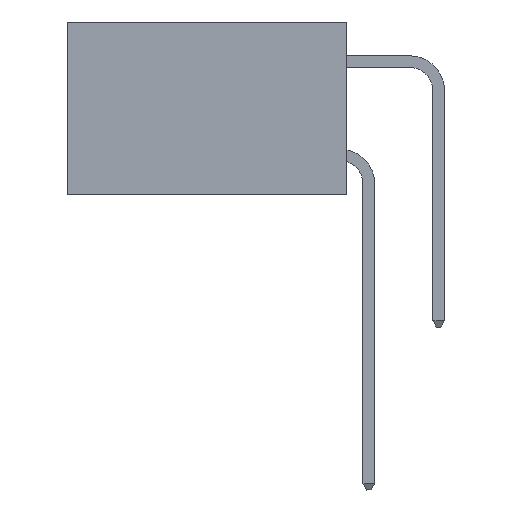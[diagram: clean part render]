
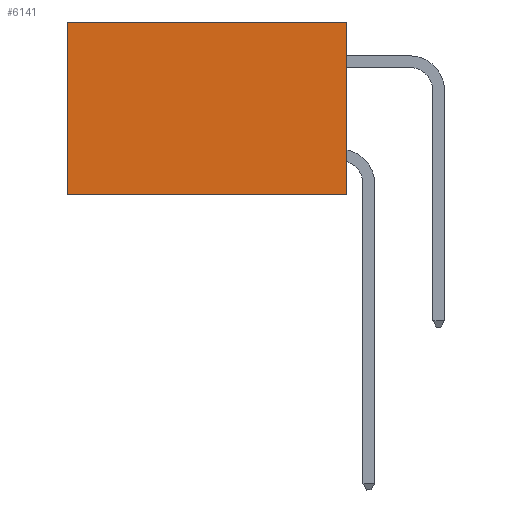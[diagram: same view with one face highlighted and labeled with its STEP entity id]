
A CAD part, left-side view. The second image highlights one B-rep face of the part: STEP entity #6141.
In plain terms, the highlighted planar face has unit normal (-1, 0, 0).
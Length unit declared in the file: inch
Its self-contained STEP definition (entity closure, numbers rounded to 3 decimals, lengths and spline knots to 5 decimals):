
#54 = DIRECTION ( 'NONE',  ( 0., 1., 0. ) ) ;
#268 = CARTESIAN_POINT ( 'NONE',  ( 0.2875, 0., 0. ) ) ;
#1064 = LINE ( 'NONE', #1661, #9241 ) ;
#1231 = AXIS2_PLACEMENT_3D ( 'NONE', #5987, #2249, #14703 ) ;
#1247 = ORIENTED_EDGE ( 'NONE', *, *, #15911, .F. ) ;
#1661 = CARTESIAN_POINT ( 'NONE',  ( 0.2875, 0., -0.37 ) ) ;
#1924 = VERTEX_POINT ( 'NONE', #8325 ) ;
#1975 = ORIENTED_EDGE ( 'NONE', *, *, #13054, .T. ) ;
#2249 = DIRECTION ( 'NONE',  ( 1., 0., 0. ) ) ;
#3926 = VERTEX_POINT ( 'NONE', #13418 ) ;
#4252 = EDGE_LOOP ( 'NONE', ( #5219, #1247, #13657, #1975 ) ) ;
#4664 = PLANE ( 'NONE',  #1231 ) ;
#4826 = EDGE_CURVE ( 'NONE', #14989, #8077, #6170, .T. ) ;
#4988 = FACE_OUTER_BOUND ( 'NONE', #4252, .T. ) ;
#5208 = EDGE_CURVE ( 'NONE', #3926, #1924, #13408, .T. ) ;
#5219 = ORIENTED_EDGE ( 'NONE', *, *, #5208, .T. ) ;
#5987 = CARTESIAN_POINT ( 'NONE',  ( 0.2875, 0., 0. ) ) ;
#6141 = ADVANCED_FACE ( 'NONE', ( #4988 ), #4664, .F. ) ;
#6170 = LINE ( 'NONE', #10400, #11237 ) ;
#6533 = DIRECTION ( 'NONE',  ( 0., 0., -1. ) ) ;
#6635 = LINE ( 'NONE', #268, #9343 ) ;
#8077 = VERTEX_POINT ( 'NONE', #12878 ) ;
#8325 = CARTESIAN_POINT ( 'NONE',  ( 0.2875, 0.6, -0.37 ) ) ;
#9241 = VECTOR ( 'NONE', #10535, 39.37008 ) ;
#9343 = VECTOR ( 'NONE', #54, 39.37008 ) ;
#10093 = VECTOR ( 'NONE', #6533, 39.37008 ) ;
#10400 = CARTESIAN_POINT ( 'NONE',  ( 0.2875, 0., 0. ) ) ;
#10535 = DIRECTION ( 'NONE',  ( 0., 1., 0. ) ) ;
#11237 = VECTOR ( 'NONE', #14216, 39.37008 ) ;
#12263 = CARTESIAN_POINT ( 'NONE',  ( 0.2875, 0., 0. ) ) ;
#12878 = CARTESIAN_POINT ( 'NONE',  ( 0.2875, 0., -0.37 ) ) ;
#13054 = EDGE_CURVE ( 'NONE', #14989, #3926, #6635, .T. ) ;
#13408 = LINE ( 'NONE', #15187, #10093 ) ;
#13418 = CARTESIAN_POINT ( 'NONE',  ( 0.2875, 0.6, 0. ) ) ;
#13657 = ORIENTED_EDGE ( 'NONE', *, *, #4826, .F. ) ;
#14216 = DIRECTION ( 'NONE',  ( 0., 0., -1. ) ) ;
#14703 = DIRECTION ( 'NONE',  ( 0., 0., -1. ) ) ;
#14989 = VERTEX_POINT ( 'NONE', #12263 ) ;
#15187 = CARTESIAN_POINT ( 'NONE',  ( 0.2875, 0.6, 0. ) ) ;
#15911 = EDGE_CURVE ( 'NONE', #8077, #1924, #1064, .T. ) ;
